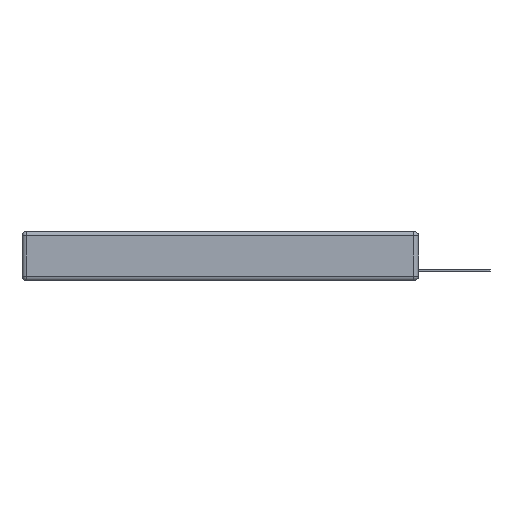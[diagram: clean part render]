
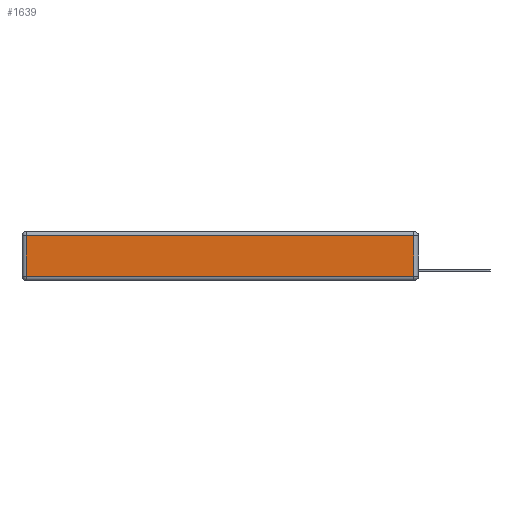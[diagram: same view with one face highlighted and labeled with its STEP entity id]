
A CAD part, left-side view. The second image highlights one B-rep face of the part: STEP entity #1639.
In plain terms, the highlighted planar face has unit normal (-1, 0, 0).
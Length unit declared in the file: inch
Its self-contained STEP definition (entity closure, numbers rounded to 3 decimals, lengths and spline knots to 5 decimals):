
#310 = CARTESIAN_POINT ( 'NONE',  ( 0., 0., -0.313 ) ) ;
#345 = LINE ( 'NONE', #5097, #2963 ) ;
#1639 = ADVANCED_FACE ( 'NONE', ( #5850 ), #8177, .T. ) ;
#1777 = VERTEX_POINT ( 'NONE', #13137 ) ;
#1934 = LINE ( 'NONE', #6685, #8406 ) ;
#2945 = CARTESIAN_POINT ( 'NONE',  ( 0., 2.72, -0.03 ) ) ;
#2963 = VECTOR ( 'NONE', #4948, 39.37008 ) ;
#3190 = DIRECTION ( 'NONE',  ( 0., 1., 0. ) ) ;
#4122 = VERTEX_POINT ( 'NONE', #8060 ) ;
#4256 = EDGE_LOOP ( 'NONE', ( #14695, #6307, #13849, #4711 ) ) ;
#4711 = ORIENTED_EDGE ( 'NONE', *, *, #14454, .T. ) ;
#4933 = CARTESIAN_POINT ( 'NONE',  ( 0., 0.03, -0.343 ) ) ;
#4948 = DIRECTION ( 'NONE',  ( 0., 0., -1. ) ) ;
#5097 = CARTESIAN_POINT ( 'NONE',  ( 0., 2.72, -0.343 ) ) ;
#5310 = EDGE_CURVE ( 'NONE', #12677, #4122, #9066, .T. ) ;
#5844 = VECTOR ( 'NONE', #13738, 39.37008 ) ;
#5850 = FACE_OUTER_BOUND ( 'NONE', #4256, .T. ) ;
#6307 = ORIENTED_EDGE ( 'NONE', *, *, #8999, .T. ) ;
#6685 = CARTESIAN_POINT ( 'NONE',  ( 0., 2.75, -0.03 ) ) ;
#7527 = CARTESIAN_POINT ( 'NONE',  ( 0., 2.72, -0.313 ) ) ;
#8060 = CARTESIAN_POINT ( 'NONE',  ( 0., 0.03, -0.313 ) ) ;
#8177 = PLANE ( 'NONE',  #14491 ) ;
#8406 = VECTOR ( 'NONE', #3190, 39.37008 ) ;
#8999 = EDGE_CURVE ( 'NONE', #4122, #1777, #9883, .T. ) ;
#9066 = LINE ( 'NONE', #310, #5844 ) ;
#9340 = DIRECTION ( 'NONE',  ( 0., 0., 1. ) ) ;
#9883 = LINE ( 'NONE', #4933, #10877 ) ;
#10476 = DIRECTION ( 'NONE',  ( -1., 0., 0. ) ) ;
#10877 = VECTOR ( 'NONE', #14338, 39.37008 ) ;
#12677 = VERTEX_POINT ( 'NONE', #7527 ) ;
#12796 = VERTEX_POINT ( 'NONE', #2945 ) ;
#13137 = CARTESIAN_POINT ( 'NONE',  ( 0., 0.03, -0.03 ) ) ;
#13738 = DIRECTION ( 'NONE',  ( 0., -1., 0. ) ) ;
#13849 = ORIENTED_EDGE ( 'NONE', *, *, #14042, .T. ) ;
#14042 = EDGE_CURVE ( 'NONE', #1777, #12796, #1934, .T. ) ;
#14164 = CARTESIAN_POINT ( 'NONE',  ( 0., 0., -0.343 ) ) ;
#14338 = DIRECTION ( 'NONE',  ( 0., 0., 1. ) ) ;
#14454 = EDGE_CURVE ( 'NONE', #12796, #12677, #345, .T. ) ;
#14491 = AXIS2_PLACEMENT_3D ( 'NONE', #14164, #10476, #9340 ) ;
#14695 = ORIENTED_EDGE ( 'NONE', *, *, #5310, .T. ) ;
